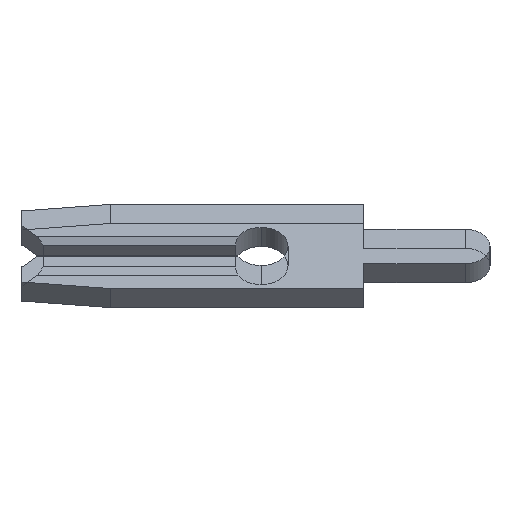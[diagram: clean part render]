
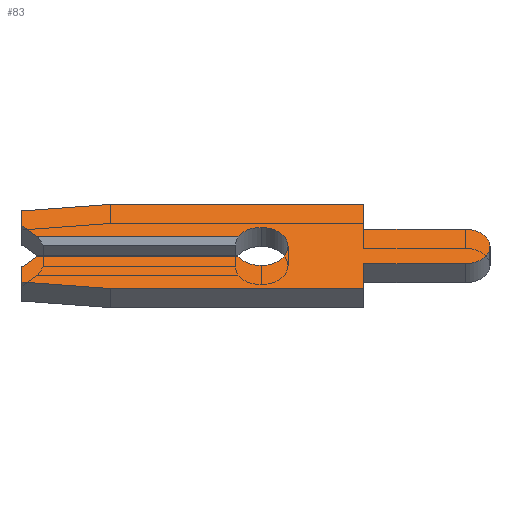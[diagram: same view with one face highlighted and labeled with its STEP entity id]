
A CAD part, left-side view. The second image highlights one B-rep face of the part: STEP entity #83.
In plain terms, the highlighted face is planar.
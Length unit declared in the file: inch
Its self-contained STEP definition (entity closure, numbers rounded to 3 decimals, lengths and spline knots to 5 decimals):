
#8 = VERTEX_POINT ( 'NONE', #2252 ) ;
#29 = EDGE_CURVE ( 'NONE', #2349, #1827, #2371, .T. ) ;
#53 = CIRCLE ( 'NONE', #391, 0.0235 ) ;
#61 = CARTESIAN_POINT ( 'NONE',  ( -0.013, 0.231, 0.028 ) ) ;
#71 = DIRECTION ( 'NONE',  ( 0., -0.995, 0.105 ) ) ;
#83 = ADVANCED_FACE ( 'NONE', ( #1975 ), #485, .F. ) ;
#112 = VECTOR ( 'NONE', #2150, 39.37008 ) ;
#134 = VECTOR ( 'NONE', #637, 39.37008 ) ;
#138 = EDGE_CURVE ( 'NONE', #1175, #2247, #1204, .T. ) ;
#169 = ORIENTED_EDGE ( 'NONE', *, *, #1525, .F. ) ;
#174 = VERTEX_POINT ( 'NONE', #1638 ) ;
#194 = EDGE_LOOP ( 'NONE', ( #680, #1731, #810, #523, #691, #2117, #460, #1280, #470, #1754, #169, #1544, #1612, #1517, #521, #239, #917, #589 ) ) ;
#235 = VECTOR ( 'NONE', #1487, 39.37008 ) ;
#239 = ORIENTED_EDGE ( 'NONE', *, *, #2145, .F. ) ;
#256 = DIRECTION ( 'NONE',  ( 0., 0., -1. ) ) ;
#268 = DIRECTION ( 'NONE',  ( 0., -1., 0. ) ) ;
#270 = VECTOR ( 'NONE', #2028, 39.37008 ) ;
#273 = VERTEX_POINT ( 'NONE', #1037 ) ;
#274 = CARTESIAN_POINT ( 'NONE',  ( -0.013, 0.216, -0.013 ) ) ;
#288 = DIRECTION ( 'NONE',  ( 0., 0., -1. ) ) ;
#293 = LINE ( 'NONE', #2243, #1626 ) ;
#299 = CARTESIAN_POINT ( 'NONE',  ( -0.013, -0.099, 0.0575 ) ) ;
#300 = VERTEX_POINT ( 'NONE', #1240 ) ;
#349 = VECTOR ( 'NONE', #464, 39.37008 ) ;
#391 = AXIS2_PLACEMENT_3D ( 'NONE', #2214, #413, #1021 ) ;
#404 = DIRECTION ( 'NONE',  ( 0., 0., -1. ) ) ;
#413 = DIRECTION ( 'NONE',  ( 1., 0., 0. ) ) ;
#415 = EDGE_CURVE ( 'NONE', #1602, #300, #775, .T. ) ;
#425 = LINE ( 'NONE', #1901, #235 ) ;
#437 = DIRECTION ( 'NONE',  ( 0., -1., 0. ) ) ;
#460 = ORIENTED_EDGE ( 'NONE', *, *, #755, .F. ) ;
#462 = DIRECTION ( 'NONE',  ( 0., 0., 1. ) ) ;
#464 = DIRECTION ( 'NONE',  ( 0., 0.707, 0.707 ) ) ;
#470 = ORIENTED_EDGE ( 'NONE', *, *, #1313, .F. ) ;
#480 = CARTESIAN_POINT ( 'NONE',  ( -0.013, 0.2105, 0.0075 ) ) ;
#485 = PLANE ( 'NONE',  #1351 ) ;
#496 = CIRCLE ( 'NONE', #639, 0.026 ) ;
#521 = ORIENTED_EDGE ( 'NONE', *, *, #138, .F. ) ;
#523 = ORIENTED_EDGE ( 'NONE', *, *, #2377, .F. ) ;
#576 = LINE ( 'NONE', #1819, #134 ) ;
#583 = AXIS2_PLACEMENT_3D ( 'NONE', #965, #1984, #404 ) ;
#589 = ORIENTED_EDGE ( 'NONE', *, *, #2061, .F. ) ;
#637 = DIRECTION ( 'NONE',  ( 0., 0., -1. ) ) ;
#639 = AXIS2_PLACEMENT_3D ( 'NONE', #2135, #1944, #949 ) ;
#680 = ORIENTED_EDGE ( 'NONE', *, *, #1891, .T. ) ;
#686 = CARTESIAN_POINT ( 'NONE',  ( -0.013, 0., 0. ) ) ;
#691 = ORIENTED_EDGE ( 'NONE', *, *, #1209, .F. ) ;
#736 = EDGE_CURVE ( 'NONE', #847, #273, #425, .T. ) ;
#755 = EDGE_CURVE ( 'NONE', #1827, #1159, #948, .T. ) ;
#775 = LINE ( 'NONE', #61, #1537 ) ;
#795 = DIRECTION ( 'NONE',  ( 0., -0.707, 0.707 ) ) ;
#810 = ORIENTED_EDGE ( 'NONE', *, *, #985, .F. ) ;
#843 = VECTOR ( 'NONE', #1890, 39.37008 ) ;
#847 = VERTEX_POINT ( 'NONE', #1108 ) ;
#872 = EDGE_CURVE ( 'NONE', #2247, #847, #1859, .T. ) ;
#893 = CARTESIAN_POINT ( 'NONE',  ( -0.013, 0.02252, 0.013 ) ) ;
#916 = VECTOR ( 'NONE', #1217, 39.37008 ) ;
#917 = ORIENTED_EDGE ( 'NONE', *, *, #415, .F. ) ;
#944 = CARTESIAN_POINT ( 'NONE',  ( -0.013, 0.231, -0.028 ) ) ;
#948 = LINE ( 'NONE', #1506, #843 ) ;
#949 = DIRECTION ( 'NONE',  ( 0., 0., -1. ) ) ;
#965 = CARTESIAN_POINT ( 'NONE',  ( -0.013, 0., 0. ) ) ;
#981 = VERTEX_POINT ( 'NONE', #1325 ) ;
#983 = CARTESIAN_POINT ( 'NONE',  ( -0.013, 0.231, 0.028 ) ) ;
#985 = EDGE_CURVE ( 'NONE', #174, #1832, #496, .T. ) ;
#1021 = DIRECTION ( 'NONE',  ( 0., 0., 1. ) ) ;
#1032 = LINE ( 'NONE', #1776, #1995 ) ;
#1037 = CARTESIAN_POINT ( 'NONE',  ( -0.013, -0.1975, 0.0235 ) ) ;
#1044 = CARTESIAN_POINT ( 'NONE',  ( -0.013, 0.146, 0.0575 ) ) ;
#1108 = CARTESIAN_POINT ( 'NONE',  ( -0.013, -0.099, 0.0235 ) ) ;
#1120 = DIRECTION ( 'NONE',  ( 0., 1., 0. ) ) ;
#1123 = CIRCLE ( 'NONE', #1249, 0.026 ) ;
#1143 = CARTESIAN_POINT ( 'NONE',  ( -0.013, 0., -0.013 ) ) ;
#1155 = LINE ( 'NONE', #1838, #2029 ) ;
#1159 = VERTEX_POINT ( 'NONE', #944 ) ;
#1175 = VERTEX_POINT ( 'NONE', #1844 ) ;
#1201 = CARTESIAN_POINT ( 'NONE',  ( -0.013, -0.099, -0.0235 ) ) ;
#1204 = LINE ( 'NONE', #1044, #2441 ) ;
#1209 = EDGE_CURVE ( 'NONE', #2129, #8, #1796, .T. ) ;
#1217 = DIRECTION ( 'NONE',  ( 0., -1., 0. ) ) ;
#1240 = CARTESIAN_POINT ( 'NONE',  ( -0.013, 0.231, 0.04857 ) ) ;
#1249 = AXIS2_PLACEMENT_3D ( 'NONE', #686, #1862, #256 ) ;
#1262 = DIRECTION ( 'NONE',  ( 0., 0., -1. ) ) ;
#1270 = VERTEX_POINT ( 'NONE', #2306 ) ;
#1280 = ORIENTED_EDGE ( 'NONE', *, *, #29, .F. ) ;
#1302 = VECTOR ( 'NONE', #288, 39.37008 ) ;
#1313 = EDGE_CURVE ( 'NONE', #1270, #2349, #1661, .T. ) ;
#1325 = CARTESIAN_POINT ( 'NONE',  ( -0.013, 0.216, 0.013 ) ) ;
#1351 = AXIS2_PLACEMENT_3D ( 'NONE', #1478, #1858, #1262 ) ;
#1454 = VERTEX_POINT ( 'NONE', #1931 ) ;
#1478 = CARTESIAN_POINT ( 'NONE',  ( -0.013, 0., 0. ) ) ;
#1487 = DIRECTION ( 'NONE',  ( 0., -1., 0. ) ) ;
#1504 = LINE ( 'NONE', #1201, #112 ) ;
#1506 = CARTESIAN_POINT ( 'NONE',  ( -0.013, 0.231, -0.028 ) ) ;
#1517 = ORIENTED_EDGE ( 'NONE', *, *, #872, .F. ) ;
#1525 = EDGE_CURVE ( 'NONE', #2047, #1454, #1504, .T. ) ;
#1537 = VECTOR ( 'NONE', #462, 39.37008 ) ;
#1544 = ORIENTED_EDGE ( 'NONE', *, *, #1920, .F. ) ;
#1602 = VERTEX_POINT ( 'NONE', #983 ) ;
#1612 = ORIENTED_EDGE ( 'NONE', *, *, #736, .F. ) ;
#1626 = VECTOR ( 'NONE', #71, 39.37008 ) ;
#1638 = CARTESIAN_POINT ( 'NONE',  ( -0.013, 0., -0.026 ) ) ;
#1658 = CARTESIAN_POINT ( 'NONE',  ( -0.013, -0.1975, -0.0235 ) ) ;
#1661 = LINE ( 'NONE', #2310, #2334 ) ;
#1731 = ORIENTED_EDGE ( 'NONE', *, *, #2005, .F. ) ;
#1751 = LINE ( 'NONE', #480, #349 ) ;
#1754 = ORIENTED_EDGE ( 'NONE', *, *, #1882, .F. ) ;
#1776 = CARTESIAN_POINT ( 'NONE',  ( -0.013, 0.2105, -0.0075 ) ) ;
#1796 = LINE ( 'NONE', #1143, #916 ) ;
#1812 = CARTESIAN_POINT ( 'NONE',  ( -0.013, 0., 0.026 ) ) ;
#1819 = CARTESIAN_POINT ( 'NONE',  ( -0.013, -0.099, -0.0575 ) ) ;
#1827 = VERTEX_POINT ( 'NONE', #2187 ) ;
#1832 = VERTEX_POINT ( 'NONE', #1812 ) ;
#1838 = CARTESIAN_POINT ( 'NONE',  ( -0.013, 0.231, 0.013 ) ) ;
#1844 = CARTESIAN_POINT ( 'NONE',  ( -0.013, 0.146, 0.0575 ) ) ;
#1858 = DIRECTION ( 'NONE',  ( 1., 0., 0. ) ) ;
#1859 = LINE ( 'NONE', #299, #1302 ) ;
#1862 = DIRECTION ( 'NONE',  ( -1., 0., 0. ) ) ;
#1882 = EDGE_CURVE ( 'NONE', #1454, #1270, #576, .T. ) ;
#1890 = DIRECTION ( 'NONE',  ( 0., 0., 1. ) ) ;
#1891 = EDGE_CURVE ( 'NONE', #981, #2224, #1155, .T. ) ;
#1901 = CARTESIAN_POINT ( 'NONE',  ( -0.013, -0.099, 0.0235 ) ) ;
#1920 = EDGE_CURVE ( 'NONE', #273, #2047, #53, .T. ) ;
#1931 = CARTESIAN_POINT ( 'NONE',  ( -0.013, -0.099, -0.0235 ) ) ;
#1944 = DIRECTION ( 'NONE',  ( -1., 0., 0. ) ) ;
#1975 = FACE_OUTER_BOUND ( 'NONE', #194, .T. ) ;
#1984 = DIRECTION ( 'NONE',  ( -1., 0., 0. ) ) ;
#1995 = VECTOR ( 'NONE', #795, 39.37008 ) ;
#2005 = EDGE_CURVE ( 'NONE', #1832, #2224, #1123, .T. ) ;
#2028 = DIRECTION ( 'NONE',  ( 0., 0.995, 0.105 ) ) ;
#2029 = VECTOR ( 'NONE', #437, 39.37008 ) ;
#2047 = VERTEX_POINT ( 'NONE', #1658 ) ;
#2061 = EDGE_CURVE ( 'NONE', #981, #1602, #1751, .T. ) ;
#2117 = ORIENTED_EDGE ( 'NONE', *, *, #2456, .F. ) ;
#2129 = VERTEX_POINT ( 'NONE', #274 ) ;
#2135 = CARTESIAN_POINT ( 'NONE',  ( -0.013, 0., 0. ) ) ;
#2145 = EDGE_CURVE ( 'NONE', #300, #1175, #293, .T. ) ;
#2150 = DIRECTION ( 'NONE',  ( 0., 1., 0. ) ) ;
#2187 = CARTESIAN_POINT ( 'NONE',  ( -0.013, 0.231, -0.04857 ) ) ;
#2214 = CARTESIAN_POINT ( 'NONE',  ( -0.013, -0.1975, 0. ) ) ;
#2224 = VERTEX_POINT ( 'NONE', #893 ) ;
#2243 = CARTESIAN_POINT ( 'NONE',  ( -0.013, 0.231, 0.04857 ) ) ;
#2247 = VERTEX_POINT ( 'NONE', #2257 ) ;
#2252 = CARTESIAN_POINT ( 'NONE',  ( -0.013, 0.02252, -0.013 ) ) ;
#2257 = CARTESIAN_POINT ( 'NONE',  ( -0.013, -0.099, 0.0575 ) ) ;
#2306 = CARTESIAN_POINT ( 'NONE',  ( -0.013, -0.099, -0.0575 ) ) ;
#2310 = CARTESIAN_POINT ( 'NONE',  ( -0.013, 0.146, -0.0575 ) ) ;
#2334 = VECTOR ( 'NONE', #1120, 39.37008 ) ;
#2349 = VERTEX_POINT ( 'NONE', #2467 ) ;
#2371 = LINE ( 'NONE', #2426, #270 ) ;
#2377 = EDGE_CURVE ( 'NONE', #8, #174, #2397, .T. ) ;
#2397 = CIRCLE ( 'NONE', #583, 0.026 ) ;
#2426 = CARTESIAN_POINT ( 'NONE',  ( -0.013, 0.231, -0.04857 ) ) ;
#2441 = VECTOR ( 'NONE', #268, 39.37008 ) ;
#2456 = EDGE_CURVE ( 'NONE', #1159, #2129, #1032, .T. ) ;
#2467 = CARTESIAN_POINT ( 'NONE',  ( -0.013, 0.146, -0.0575 ) ) ;
